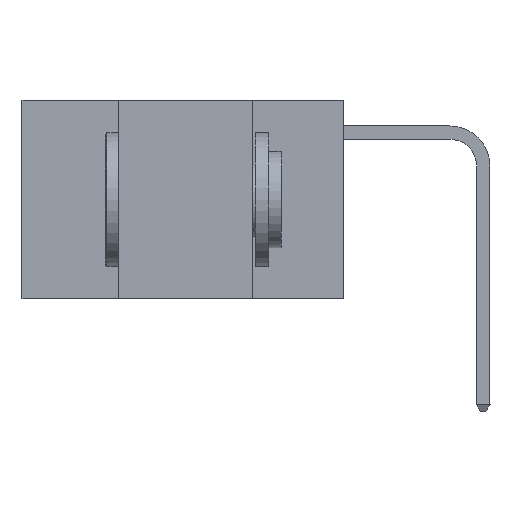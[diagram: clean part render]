
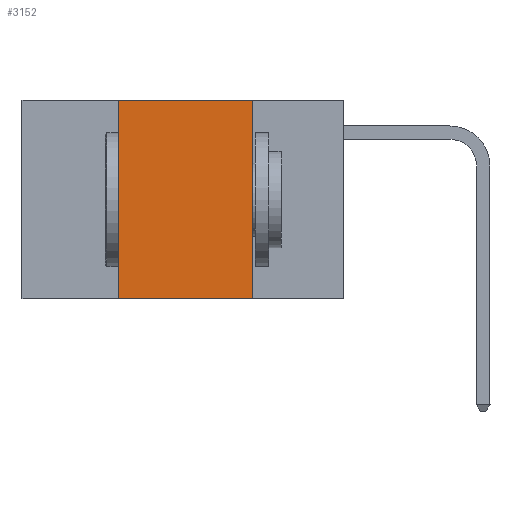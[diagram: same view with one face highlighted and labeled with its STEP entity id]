
A CAD part, left-side view. The second image highlights one B-rep face of the part: STEP entity #3152.
In plain terms, the highlighted planar face has unit normal (-1, 0, 0).
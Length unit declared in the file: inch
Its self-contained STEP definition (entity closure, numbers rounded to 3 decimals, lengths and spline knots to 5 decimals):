
#260 = VERTEX_POINT ( 'NONE', #822 ) ;
#413 = ORIENTED_EDGE ( 'NONE', *, *, #6240, .F. ) ;
#457 = ORIENTED_EDGE ( 'NONE', *, *, #2149, .F. ) ;
#518 = ORIENTED_EDGE ( 'NONE', *, *, #7152, .F. ) ;
#543 = ORIENTED_EDGE ( 'NONE', *, *, #1902, .T. ) ;
#822 = CARTESIAN_POINT ( 'NONE',  ( 0., 0.42, -0.37 ) ) ;
#1306 = VERTEX_POINT ( 'NONE', #2476 ) ;
#1720 = DIRECTION ( 'NONE',  ( 0., 0., -1. ) ) ;
#1902 = EDGE_CURVE ( 'NONE', #260, #2273, #5091, .T. ) ;
#2149 = EDGE_CURVE ( 'NONE', #1306, #4844, #5659, .T. ) ;
#2273 = VERTEX_POINT ( 'NONE', #4475 ) ;
#2476 = CARTESIAN_POINT ( 'NONE',  ( 0., 0.42, 0. ) ) ;
#2749 = AXIS2_PLACEMENT_3D ( 'NONE', #5596, #3986, #3931 ) ;
#3152 = ADVANCED_FACE ( 'NONE', ( #6582 ), #6900, .F. ) ;
#3931 = DIRECTION ( 'NONE',  ( 0., 0., -1. ) ) ;
#3986 = DIRECTION ( 'NONE',  ( 1., 0., 0. ) ) ;
#4475 = CARTESIAN_POINT ( 'NONE',  ( 0., 0.17, -0.37 ) ) ;
#4844 = VERTEX_POINT ( 'NONE', #5350 ) ;
#4885 = VECTOR ( 'NONE', #7542, 39.37008 ) ;
#5091 = LINE ( 'NONE', #7526, #4885 ) ;
#5237 = DIRECTION ( 'NONE',  ( 0., -1., 0. ) ) ;
#5350 = CARTESIAN_POINT ( 'NONE',  ( 0., 0.17, 0. ) ) ;
#5396 = LINE ( 'NONE', #7945, #8393 ) ;
#5596 = CARTESIAN_POINT ( 'NONE',  ( 0., 0.6, 0. ) ) ;
#5659 = LINE ( 'NONE', #8562, #6683 ) ;
#6240 = EDGE_CURVE ( 'NONE', #4844, #2273, #6804, .T. ) ;
#6246 = VECTOR ( 'NONE', #1720, 39.37008 ) ;
#6582 = FACE_OUTER_BOUND ( 'NONE', #7576, .T. ) ;
#6683 = VECTOR ( 'NONE', #5237, 39.37008 ) ;
#6804 = LINE ( 'NONE', #8388, #6246 ) ;
#6900 = PLANE ( 'NONE',  #2749 ) ;
#7152 = EDGE_CURVE ( 'NONE', #260, #1306, #5396, .T. ) ;
#7526 = CARTESIAN_POINT ( 'NONE',  ( 0., 0.6, -0.37 ) ) ;
#7542 = DIRECTION ( 'NONE',  ( 0., -1., 0. ) ) ;
#7576 = EDGE_LOOP ( 'NONE', ( #413, #457, #518, #543 ) ) ;
#7945 = CARTESIAN_POINT ( 'NONE',  ( 0., 0.42, 0. ) ) ;
#8388 = CARTESIAN_POINT ( 'NONE',  ( 0., 0.17, 0. ) ) ;
#8393 = VECTOR ( 'NONE', #8533, 39.37008 ) ;
#8533 = DIRECTION ( 'NONE',  ( 0., 0., 1. ) ) ;
#8562 = CARTESIAN_POINT ( 'NONE',  ( 0., 0.6, 0. ) ) ;
